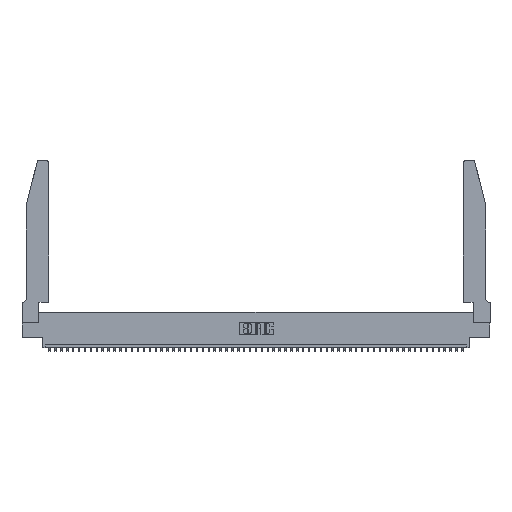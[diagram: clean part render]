
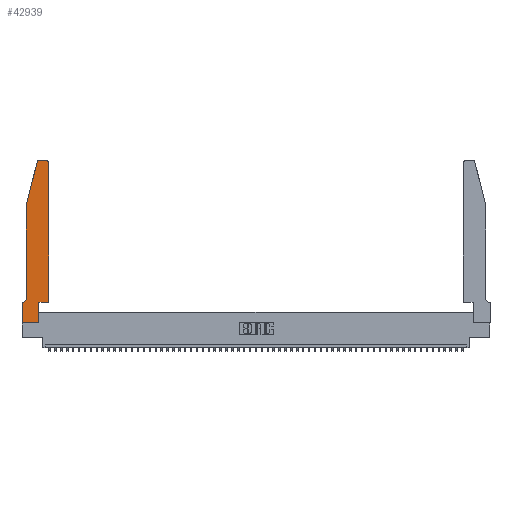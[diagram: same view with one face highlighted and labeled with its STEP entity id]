
A CAD part, top view. The second image highlights one B-rep face of the part: STEP entity #42939.
In plain terms, the highlighted planar face has unit normal (0, 0, 1).
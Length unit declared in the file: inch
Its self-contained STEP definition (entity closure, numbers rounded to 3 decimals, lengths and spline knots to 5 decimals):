
#190 = EDGE_CURVE ( 'NONE', #5913, #14268, #15179, .T. ) ;
#1177 = CARTESIAN_POINT ( 'NONE',  ( 0.0755, 0.42, 0.37 ) ) ;
#1792 = LINE ( 'NONE', #4529, #45352 ) ;
#2117 = ORIENTED_EDGE ( 'NONE', *, *, #42068, .T. ) ;
#2533 = EDGE_CURVE ( 'NONE', #32327, #12420, #27979, .T. ) ;
#2887 = VECTOR ( 'NONE', #9262, 39.37008 ) ;
#4529 = CARTESIAN_POINT ( 'NONE',  ( 0.4505, 0.35, 0.37 ) ) ;
#4566 = CARTESIAN_POINT ( 'NONE',  ( 0., 0., 0.37 ) ) ;
#5895 = DIRECTION ( 'NONE',  ( -1., 0., 0. ) ) ;
#5913 = VERTEX_POINT ( 'NONE', #42015 ) ;
#6279 = LINE ( 'NONE', #12356, #30534 ) ;
#6602 = VERTEX_POINT ( 'NONE', #23354 ) ;
#6803 = EDGE_CURVE ( 'NONE', #43756, #32327, #16989, .T. ) ;
#7032 = ORIENTED_EDGE ( 'NONE', *, *, #52859, .T. ) ;
#7524 = VECTOR ( 'NONE', #30254, 39.37008 ) ;
#8429 = AXIS2_PLACEMENT_3D ( 'NONE', #26209, #9459, #51504 ) ;
#8984 = CARTESIAN_POINT ( 'NONE',  ( 0., 0.35, 0.37 ) ) ;
#9262 = DIRECTION ( 'NONE',  ( 1., 0., 0. ) ) ;
#9459 = DIRECTION ( 'NONE',  ( 0., 0., -1. ) ) ;
#10356 = VECTOR ( 'NONE', #45832, 39.37008 ) ;
#10591 = FACE_OUTER_BOUND ( 'NONE', #33742, .T. ) ;
#11106 = LINE ( 'NONE', #41695, #43173 ) ;
#11158 = CARTESIAN_POINT ( 'NONE',  ( 0.0055, 0.35, 0.37 ) ) ;
#11589 = DIRECTION ( 'NONE',  ( 0., 0., 1. ) ) ;
#11650 = VECTOR ( 'NONE', #29781, 39.37008 ) ;
#12222 = DIRECTION ( 'NONE',  ( -1., 0., 0. ) ) ;
#12333 = ORIENTED_EDGE ( 'NONE', *, *, #17661, .T. ) ;
#12356 = CARTESIAN_POINT ( 'NONE',  ( 0.4505, 0.35, 0.37 ) ) ;
#12420 = VERTEX_POINT ( 'NONE', #37182 ) ;
#13027 = CARTESIAN_POINT ( 'NONE',  ( 0.4505, 0.35, 0.37 ) ) ;
#13342 = CARTESIAN_POINT ( 'NONE',  ( 0., 0., 0.37 ) ) ;
#13640 = LINE ( 'NONE', #32802, #10356 ) ;
#14248 = VECTOR ( 'NONE', #48593, 39.37008 ) ;
#14261 = DIRECTION ( 'NONE',  ( 1., 0., 0. ) ) ;
#14268 = VERTEX_POINT ( 'NONE', #40181 ) ;
#14463 = ORIENTED_EDGE ( 'NONE', *, *, #54103, .T. ) ;
#15179 = CIRCLE ( 'NONE', #38077, 0.03 ) ;
#15759 = EDGE_CURVE ( 'NONE', #14268, #28836, #11106, .T. ) ;
#16095 = LINE ( 'NONE', #39208, #7524 ) ;
#16989 = LINE ( 'NONE', #38142, #14248 ) ;
#17069 = ORIENTED_EDGE ( 'NONE', *, *, #15759, .T. ) ;
#17661 = EDGE_CURVE ( 'NONE', #21846, #5913, #6279, .T. ) ;
#18220 = DIRECTION ( 'NONE',  ( 1., 0., 0. ) ) ;
#20044 = DIRECTION ( 'NONE',  ( 0., 0., 1. ) ) ;
#21846 = VERTEX_POINT ( 'NONE', #13027 ) ;
#22336 = CARTESIAN_POINT ( 'NONE',  ( 0.284, 2.72, 0.37 ) ) ;
#23116 = DIRECTION ( 'NONE',  ( 0., 0., 1. ) ) ;
#23354 = CARTESIAN_POINT ( 'NONE',  ( 0.25487, 2.72718, 0.37 ) ) ;
#23533 = ORIENTED_EDGE ( 'NONE', *, *, #35899, .T. ) ;
#24091 = VERTEX_POINT ( 'NONE', #11158 ) ;
#25359 = DIRECTION ( 'NONE',  ( 0., 1., 0. ) ) ;
#25456 = CARTESIAN_POINT ( 'NONE',  ( 0.2865, 0.35, 0.37 ) ) ;
#25595 = EDGE_CURVE ( 'NONE', #51321, #24091, #37569, .T. ) ;
#26209 = CARTESIAN_POINT ( 'NONE',  ( 0.0055, 0.42, 0.37 ) ) ;
#27607 = VERTEX_POINT ( 'NONE', #39018 ) ;
#27979 = LINE ( 'NONE', #13342, #2887 ) ;
#28295 = CARTESIAN_POINT ( 'NONE',  ( 0.4205, 2.72, 0.37 ) ) ;
#28836 = VERTEX_POINT ( 'NONE', #48415 ) ;
#29332 = LINE ( 'NONE', #25456, #11650 ) ;
#29781 = DIRECTION ( 'NONE',  ( 0., 1., 0. ) ) ;
#29926 = ORIENTED_EDGE ( 'NONE', *, *, #25595, .T. ) ;
#30254 = DIRECTION ( 'NONE',  ( 0., -1., 0. ) ) ;
#30534 = VECTOR ( 'NONE', #25359, 39.37008 ) ;
#32327 = VERTEX_POINT ( 'NONE', #4566 ) ;
#32802 = CARTESIAN_POINT ( 'NONE',  ( 0.0755, 2., 0.37 ) ) ;
#33742 = EDGE_LOOP ( 'NONE', ( #17069, #33855, #7032, #2117, #29926, #23533, #53238, #47004, #14463, #35544, #12333, #42040 ) ) ;
#33855 = ORIENTED_EDGE ( 'NONE', *, *, #38103, .T. ) ;
#35544 = ORIENTED_EDGE ( 'NONE', *, *, #38728, .T. ) ;
#35899 = EDGE_CURVE ( 'NONE', #24091, #43756, #51422, .T. ) ;
#36883 = DIRECTION ( 'NONE',  ( 1., 0., 0. ) ) ;
#37182 = CARTESIAN_POINT ( 'NONE',  ( 0.2865, 0., 0.37 ) ) ;
#37569 = CIRCLE ( 'NONE', #8429, 0.07 ) ;
#38077 = AXIS2_PLACEMENT_3D ( 'NONE', #28295, #11589, #36883 ) ;
#38103 = EDGE_CURVE ( 'NONE', #28836, #6602, #43301, .T. ) ;
#38142 = CARTESIAN_POINT ( 'NONE',  ( 0., 0., 0.37 ) ) ;
#38728 = EDGE_CURVE ( 'NONE', #54328, #21846, #1792, .T. ) ;
#38932 = VECTOR ( 'NONE', #5895, 39.37008 ) ;
#39018 = CARTESIAN_POINT ( 'NONE',  ( 0.0755, 2., 0.37 ) ) ;
#39208 = CARTESIAN_POINT ( 'NONE',  ( 0.0755, 2., 0.37 ) ) ;
#39598 = CARTESIAN_POINT ( 'NONE',  ( 0.2865, 0.35, 0.37 ) ) ;
#39710 = CARTESIAN_POINT ( 'NONE',  ( 0.0755, 0.35, 0.37 ) ) ;
#40181 = CARTESIAN_POINT ( 'NONE',  ( 0.4205, 2.75, 0.37 ) ) ;
#40705 = PLANE ( 'NONE',  #42303 ) ;
#41695 = CARTESIAN_POINT ( 'NONE',  ( 0.2605, 2.75, 0.37 ) ) ;
#42015 = CARTESIAN_POINT ( 'NONE',  ( 0.4505, 2.72, 0.37 ) ) ;
#42040 = ORIENTED_EDGE ( 'NONE', *, *, #190, .T. ) ;
#42068 = EDGE_CURVE ( 'NONE', #27607, #51321, #16095, .T. ) ;
#42303 = AXIS2_PLACEMENT_3D ( 'NONE', #53500, #20044, #53884 ) ;
#42939 = ADVANCED_FACE ( 'NONE', ( #10591 ), #40705, .T. ) ;
#43173 = VECTOR ( 'NONE', #12222, 39.37008 ) ;
#43301 = CIRCLE ( 'NONE', #45760, 0.03 ) ;
#43756 = VERTEX_POINT ( 'NONE', #8984 ) ;
#45352 = VECTOR ( 'NONE', #18220, 39.37008 ) ;
#45760 = AXIS2_PLACEMENT_3D ( 'NONE', #22336, #23116, #14261 ) ;
#45832 = DIRECTION ( 'NONE',  ( -0.239, -0.971, 0. ) ) ;
#47004 = ORIENTED_EDGE ( 'NONE', *, *, #2533, .T. ) ;
#48415 = CARTESIAN_POINT ( 'NONE',  ( 0.284, 2.75, 0.37 ) ) ;
#48593 = DIRECTION ( 'NONE',  ( 0., -1., 0. ) ) ;
#51321 = VERTEX_POINT ( 'NONE', #1177 ) ;
#51422 = LINE ( 'NONE', #39710, #38932 ) ;
#51504 = DIRECTION ( 'NONE',  ( -1., 0., 0. ) ) ;
#52859 = EDGE_CURVE ( 'NONE', #6602, #27607, #13640, .T. ) ;
#53238 = ORIENTED_EDGE ( 'NONE', *, *, #6803, .T. ) ;
#53500 = CARTESIAN_POINT ( 'NONE',  ( 0., 0.35, 0.37 ) ) ;
#53884 = DIRECTION ( 'NONE',  ( 1., 0., 0. ) ) ;
#54103 = EDGE_CURVE ( 'NONE', #12420, #54328, #29332, .T. ) ;
#54328 = VERTEX_POINT ( 'NONE', #39598 ) ;
